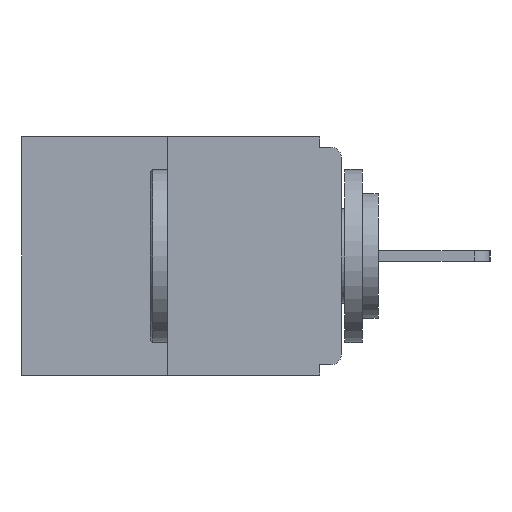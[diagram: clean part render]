
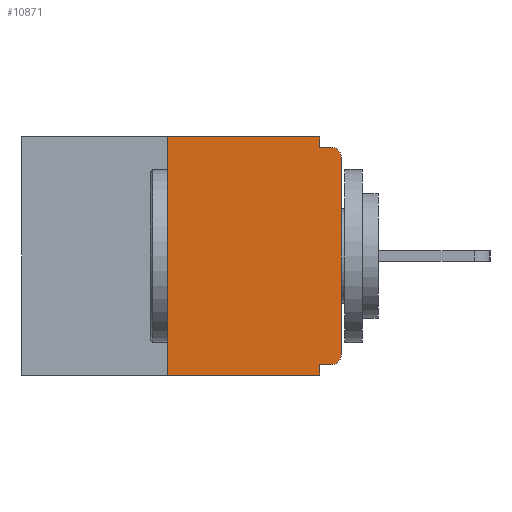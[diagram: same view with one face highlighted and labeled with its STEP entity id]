
A CAD part, left-side view. The second image highlights one B-rep face of the part: STEP entity #10871.
In plain terms, the highlighted planar face has unit normal (-1, 0, 0).
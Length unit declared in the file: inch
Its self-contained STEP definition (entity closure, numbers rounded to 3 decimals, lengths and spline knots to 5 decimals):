
#72 = VERTEX_POINT ( 'NONE', #16030 ) ;
#381 = DIRECTION ( 'NONE',  ( 0., 1., 0. ) ) ;
#569 = VERTEX_POINT ( 'NONE', #20527 ) ;
#1475 = ORIENTED_EDGE ( 'NONE', *, *, #12250, .T. ) ;
#1639 = EDGE_LOOP ( 'NONE', ( #19159, #7989, #21276, #12297, #7202, #8362, #1475, #7907, #13106, #19446 ) ) ;
#2056 = LINE ( 'NONE', #14074, #10188 ) ;
#2299 = CARTESIAN_POINT ( 'NONE',  ( 0., 0.015, -0.015 ) ) ;
#2486 = DIRECTION ( 'NONE',  ( 0., 0., -1. ) ) ;
#3174 = VECTOR ( 'NONE', #381, 39.37008 ) ;
#3216 = CARTESIAN_POINT ( 'NONE',  ( 0., 0.015, -0.03 ) ) ;
#3263 = EDGE_CURVE ( 'NONE', #14113, #23344, #10726, .T. ) ;
#3447 = CARTESIAN_POINT ( 'NONE',  ( 0., 0.015, -0.328 ) ) ;
#3665 = AXIS2_PLACEMENT_3D ( 'NONE', #3216, #5295, #18002 ) ;
#4648 = DIRECTION ( 'NONE',  ( 0., 0., 1. ) ) ;
#5295 = DIRECTION ( 'NONE',  ( -1., 0., 0. ) ) ;
#5360 = VERTEX_POINT ( 'NONE', #16171 ) ;
#5667 = DIRECTION ( 'NONE',  ( 1., 0., 0. ) ) ;
#5927 = VERTEX_POINT ( 'NONE', #2299 ) ;
#6122 = FACE_OUTER_BOUND ( 'NONE', #1639, .T. ) ;
#6270 = CARTESIAN_POINT ( 'NONE',  ( 0., 0.031, 0. ) ) ;
#6535 = VERTEX_POINT ( 'NONE', #19914 ) ;
#6691 = VECTOR ( 'NONE', #4648, 39.37008 ) ;
#7082 = LINE ( 'NONE', #13743, #13137 ) ;
#7202 = ORIENTED_EDGE ( 'NONE', *, *, #3263, .F. ) ;
#7376 = AXIS2_PLACEMENT_3D ( 'NONE', #17544, #17390, #10297 ) ;
#7487 = LINE ( 'NONE', #18132, #19992 ) ;
#7907 = ORIENTED_EDGE ( 'NONE', *, *, #18651, .T. ) ;
#7989 = ORIENTED_EDGE ( 'NONE', *, *, #23823, .F. ) ;
#8362 = ORIENTED_EDGE ( 'NONE', *, *, #17201, .T. ) ;
#8506 = AXIS2_PLACEMENT_3D ( 'NONE', #12981, #5667, #11372 ) ;
#8531 = CARTESIAN_POINT ( 'NONE',  ( 0., 0.25, 0. ) ) ;
#8759 = LINE ( 'NONE', #8876, #13929 ) ;
#8876 = CARTESIAN_POINT ( 'NONE',  ( 0., 0.46, 0. ) ) ;
#9340 = CARTESIAN_POINT ( 'NONE',  ( 0., 0.031, -0.343 ) ) ;
#9945 = CARTESIAN_POINT ( 'NONE',  ( 0., 0.25, -0.343 ) ) ;
#10116 = EDGE_CURVE ( 'NONE', #72, #569, #8759, .T. ) ;
#10188 = VECTOR ( 'NONE', #21691, 39.37008 ) ;
#10251 = EDGE_CURVE ( 'NONE', #16655, #5927, #2056, .T. ) ;
#10297 = DIRECTION ( 'NONE',  ( 0., 0., -1. ) ) ;
#10572 = CIRCLE ( 'NONE', #7376, 0.015 ) ;
#10726 = LINE ( 'NONE', #13441, #3174 ) ;
#10871 = ADVANCED_FACE ( 'NONE', ( #6122 ), #14959, .F. ) ;
#11372 = DIRECTION ( 'NONE',  ( 0., 0., -1. ) ) ;
#12250 = EDGE_CURVE ( 'NONE', #6535, #5360, #21547, .T. ) ;
#12281 = CARTESIAN_POINT ( 'NONE',  ( 0., 0.031, -0.015 ) ) ;
#12297 = ORIENTED_EDGE ( 'NONE', *, *, #14913, .F. ) ;
#12402 = CARTESIAN_POINT ( 'NONE',  ( 0., 0., 0. ) ) ;
#12981 = CARTESIAN_POINT ( 'NONE',  ( 0., 0.46, 0. ) ) ;
#13106 = ORIENTED_EDGE ( 'NONE', *, *, #10251, .F. ) ;
#13137 = VECTOR ( 'NONE', #2486, 39.37008 ) ;
#13441 = CARTESIAN_POINT ( 'NONE',  ( 0., 0., -0.328 ) ) ;
#13743 = CARTESIAN_POINT ( 'NONE',  ( 0., 0.031, -0.343 ) ) ;
#13803 = VERTEX_POINT ( 'NONE', #9945 ) ;
#13916 = LINE ( 'NONE', #8531, #6691 ) ;
#13929 = VECTOR ( 'NONE', #18626, 39.37008 ) ;
#14074 = CARTESIAN_POINT ( 'NONE',  ( 0., 0., -0.015 ) ) ;
#14113 = VERTEX_POINT ( 'NONE', #3447 ) ;
#14913 = EDGE_CURVE ( 'NONE', #23344, #16193, #7082, .T. ) ;
#14959 = PLANE ( 'NONE',  #8506 ) ;
#15385 = EDGE_CURVE ( 'NONE', #13803, #16193, #7487, .T. ) ;
#15964 = DIRECTION ( 'NONE',  ( 0., -1., 0. ) ) ;
#16030 = CARTESIAN_POINT ( 'NONE',  ( 0., 0.25, 0. ) ) ;
#16102 = DIRECTION ( 'NONE',  ( 0., 0., 1. ) ) ;
#16171 = CARTESIAN_POINT ( 'NONE',  ( 0., 0., -0.03 ) ) ;
#16193 = VERTEX_POINT ( 'NONE', #9340 ) ;
#16655 = VERTEX_POINT ( 'NONE', #12281 ) ;
#17201 = EDGE_CURVE ( 'NONE', #14113, #6535, #10572, .T. ) ;
#17277 = EDGE_CURVE ( 'NONE', #569, #16655, #19321, .T. ) ;
#17390 = DIRECTION ( 'NONE',  ( -1., 0., 0. ) ) ;
#17544 = CARTESIAN_POINT ( 'NONE',  ( 0., 0.015, -0.313 ) ) ;
#18002 = DIRECTION ( 'NONE',  ( 0., 0., -1. ) ) ;
#18132 = CARTESIAN_POINT ( 'NONE',  ( 0., 0.46, -0.343 ) ) ;
#18205 = CIRCLE ( 'NONE', #3665, 0.015 ) ;
#18612 = VECTOR ( 'NONE', #16102, 39.37008 ) ;
#18626 = DIRECTION ( 'NONE',  ( 0., -1., 0. ) ) ;
#18651 = EDGE_CURVE ( 'NONE', #5360, #5927, #18205, .T. ) ;
#19159 = ORIENTED_EDGE ( 'NONE', *, *, #10116, .F. ) ;
#19321 = LINE ( 'NONE', #6270, #19891 ) ;
#19343 = DIRECTION ( 'NONE',  ( 0., 0., -1. ) ) ;
#19446 = ORIENTED_EDGE ( 'NONE', *, *, #17277, .F. ) ;
#19891 = VECTOR ( 'NONE', #19343, 39.37008 ) ;
#19914 = CARTESIAN_POINT ( 'NONE',  ( 0., 0., -0.313 ) ) ;
#19992 = VECTOR ( 'NONE', #15964, 39.37008 ) ;
#20527 = CARTESIAN_POINT ( 'NONE',  ( 0., 0.031, 0. ) ) ;
#21276 = ORIENTED_EDGE ( 'NONE', *, *, #15385, .T. ) ;
#21547 = LINE ( 'NONE', #12402, #18612 ) ;
#21691 = DIRECTION ( 'NONE',  ( 0., -1., 0. ) ) ;
#23344 = VERTEX_POINT ( 'NONE', #24030 ) ;
#23823 = EDGE_CURVE ( 'NONE', #13803, #72, #13916, .T. ) ;
#24030 = CARTESIAN_POINT ( 'NONE',  ( 0., 0.031, -0.328 ) ) ;
